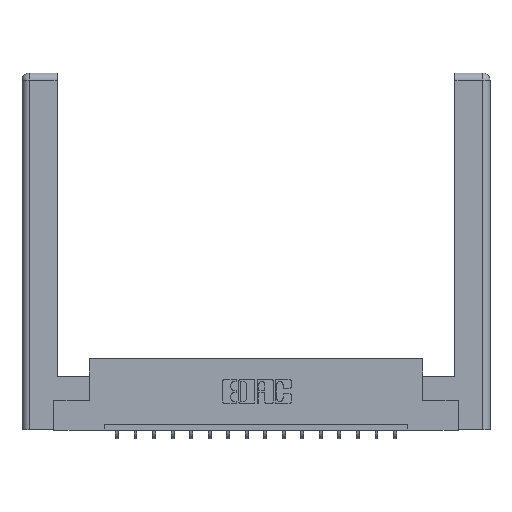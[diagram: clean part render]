
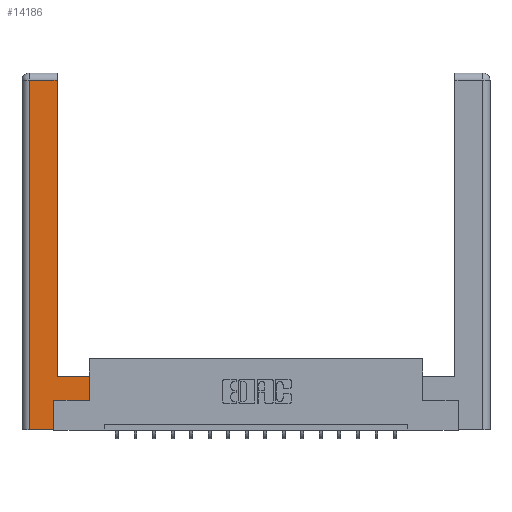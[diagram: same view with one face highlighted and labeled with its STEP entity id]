
A CAD part, top view. The second image highlights one B-rep face of the part: STEP entity #14186.
In plain terms, the highlighted planar face has unit normal (0, 0, 1).
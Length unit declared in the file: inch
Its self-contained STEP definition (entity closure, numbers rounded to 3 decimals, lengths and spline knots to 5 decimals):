
#124 = LINE ( 'NONE', #9263, #10130 ) ;
#173 = LINE ( 'NONE', #6922, #4307 ) ;
#580 = VERTEX_POINT ( 'NONE', #914 ) ;
#897 = ORIENTED_EDGE ( 'NONE', *, *, #12942, .T. ) ;
#914 = CARTESIAN_POINT ( 'NONE',  ( 0.265, 0., 0. ) ) ;
#1389 = EDGE_CURVE ( 'NONE', #9377, #4753, #7850, .T. ) ;
#1452 = CARTESIAN_POINT ( 'NONE',  ( 0.565, 0.245, 0. ) ) ;
#1909 = ORIENTED_EDGE ( 'NONE', *, *, #1389, .T. ) ;
#2461 = VECTOR ( 'NONE', #6935, 39.37008 ) ;
#2793 = EDGE_CURVE ( 'NONE', #9331, #9377, #6300, .T. ) ;
#3086 = ORIENTED_EDGE ( 'NONE', *, *, #5453, .T. ) ;
#3210 = VECTOR ( 'NONE', #15372, 39.37008 ) ;
#3735 = EDGE_CURVE ( 'NONE', #580, #17538, #5476, .T. ) ;
#4129 = CARTESIAN_POINT ( 'NONE',  ( 0.265, 0.245, 0. ) ) ;
#4307 = VECTOR ( 'NONE', #10786, 39.37008 ) ;
#4323 = DIRECTION ( 'NONE',  ( -1., 0., 0. ) ) ;
#4338 = CARTESIAN_POINT ( 'NONE',  ( 0.0615, 0., 0. ) ) ;
#4398 = CARTESIAN_POINT ( 'NONE',  ( 0.565, 0.245, 0. ) ) ;
#4753 = VERTEX_POINT ( 'NONE', #13245 ) ;
#5428 = CARTESIAN_POINT ( 'NONE',  ( 0.565, 0.45, 0. ) ) ;
#5453 = EDGE_CURVE ( 'NONE', #6095, #580, #173, .T. ) ;
#5476 = LINE ( 'NONE', #13789, #15887 ) ;
#5578 = VERTEX_POINT ( 'NONE', #1452 ) ;
#5622 = EDGE_CURVE ( 'NONE', #4753, #5787, #6946, .T. ) ;
#5787 = VERTEX_POINT ( 'NONE', #12718 ) ;
#5957 = CARTESIAN_POINT ( 'NONE',  ( 0., 0., 0. ) ) ;
#6095 = VERTEX_POINT ( 'NONE', #4338 ) ;
#6300 = LINE ( 'NONE', #7083, #17577 ) ;
#6922 = CARTESIAN_POINT ( 'NONE',  ( 0.265, 0., 0. ) ) ;
#6935 = DIRECTION ( 'NONE',  ( 0., 1., 0. ) ) ;
#6946 = LINE ( 'NONE', #7087, #3210 ) ;
#7083 = CARTESIAN_POINT ( 'NONE',  ( 0.295, 0.45, 0. ) ) ;
#7087 = CARTESIAN_POINT ( 'NONE',  ( 0.0615, 2.94, 0. ) ) ;
#7101 = ORIENTED_EDGE ( 'NONE', *, *, #10411, .T. ) ;
#7575 = EDGE_LOOP ( 'NONE', ( #1909, #17340, #7101, #3086, #10448, #897, #12493, #15829 ) ) ;
#7850 = LINE ( 'NONE', #12197, #10646 ) ;
#8294 = DIRECTION ( 'NONE',  ( 0., 1., 0. ) ) ;
#8684 = DIRECTION ( 'NONE',  ( -1., 0., 0. ) ) ;
#8737 = DIRECTION ( 'NONE',  ( 0., 0., -1. ) ) ;
#9201 = DIRECTION ( 'NONE',  ( 0., -1., 0. ) ) ;
#9263 = CARTESIAN_POINT ( 'NONE',  ( 0.0615, 0., 0. ) ) ;
#9331 = VERTEX_POINT ( 'NONE', #5428 ) ;
#9377 = VERTEX_POINT ( 'NONE', #10928 ) ;
#9918 = AXIS2_PLACEMENT_3D ( 'NONE', #5957, #8737, #8684 ) ;
#10130 = VECTOR ( 'NONE', #9201, 39.37008 ) ;
#10411 = EDGE_CURVE ( 'NONE', #5787, #6095, #124, .T. ) ;
#10448 = ORIENTED_EDGE ( 'NONE', *, *, #3735, .T. ) ;
#10646 = VECTOR ( 'NONE', #13468, 39.37008 ) ;
#10786 = DIRECTION ( 'NONE',  ( 1., 0., 0. ) ) ;
#10908 = LINE ( 'NONE', #4398, #11557 ) ;
#10928 = CARTESIAN_POINT ( 'NONE',  ( 0.295, 0.45, 0. ) ) ;
#10952 = LINE ( 'NONE', #12318, #2461 ) ;
#11557 = VECTOR ( 'NONE', #14110, 39.37008 ) ;
#11583 = PLANE ( 'NONE',  #9918 ) ;
#12197 = CARTESIAN_POINT ( 'NONE',  ( 0.295, 3., 0. ) ) ;
#12318 = CARTESIAN_POINT ( 'NONE',  ( 0.565, 0.45, 0. ) ) ;
#12493 = ORIENTED_EDGE ( 'NONE', *, *, #16113, .T. ) ;
#12718 = CARTESIAN_POINT ( 'NONE',  ( 0.0615, 2.94, 0. ) ) ;
#12942 = EDGE_CURVE ( 'NONE', #17538, #5578, #10908, .T. ) ;
#13245 = CARTESIAN_POINT ( 'NONE',  ( 0.295, 2.94, 0. ) ) ;
#13468 = DIRECTION ( 'NONE',  ( 0., 1., 0. ) ) ;
#13789 = CARTESIAN_POINT ( 'NONE',  ( 0.265, 0.245, 0. ) ) ;
#14110 = DIRECTION ( 'NONE',  ( 1., 0., 0. ) ) ;
#14186 = ADVANCED_FACE ( 'NONE', ( #15646 ), #11583, .F. ) ;
#15372 = DIRECTION ( 'NONE',  ( -1., 0., 0. ) ) ;
#15646 = FACE_OUTER_BOUND ( 'NONE', #7575, .T. ) ;
#15829 = ORIENTED_EDGE ( 'NONE', *, *, #2793, .T. ) ;
#15887 = VECTOR ( 'NONE', #8294, 39.37008 ) ;
#16113 = EDGE_CURVE ( 'NONE', #5578, #9331, #10952, .T. ) ;
#17340 = ORIENTED_EDGE ( 'NONE', *, *, #5622, .T. ) ;
#17538 = VERTEX_POINT ( 'NONE', #4129 ) ;
#17577 = VECTOR ( 'NONE', #4323, 39.37008 ) ;
